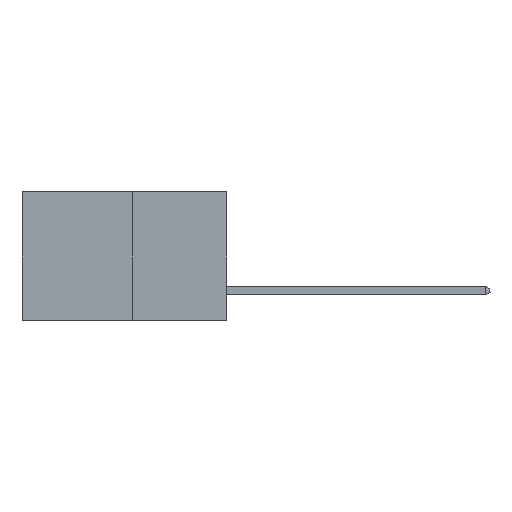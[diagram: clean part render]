
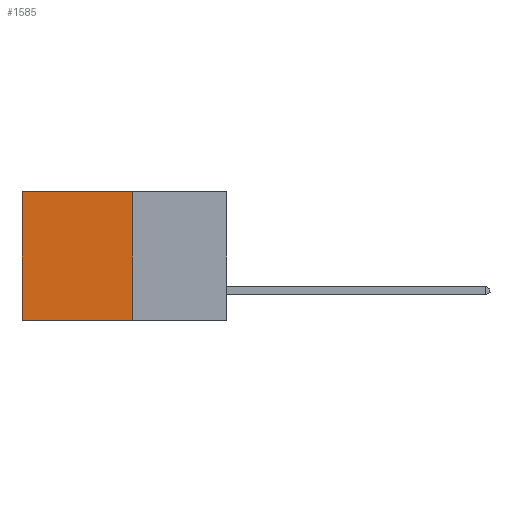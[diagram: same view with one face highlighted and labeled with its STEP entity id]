
A CAD part, left-side view. The second image highlights one B-rep face of the part: STEP entity #1585.
In plain terms, the highlighted planar face has unit normal (-1, 0, 0).
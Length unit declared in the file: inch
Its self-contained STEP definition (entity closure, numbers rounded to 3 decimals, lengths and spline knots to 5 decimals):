
#1541 = VERTEX_POINT ( 'NONE', #22558 ) ;
#1585 = ADVANCED_FACE ( 'NONE', ( #32372 ), #22675, .F. ) ;
#1615 = DIRECTION ( 'NONE',  ( 0., 0., -1. ) ) ;
#1715 = CARTESIAN_POINT ( 'NONE',  ( 0.277, 0.27, -0.37 ) ) ;
#4461 = VECTOR ( 'NONE', #7080, 39.37008 ) ;
#4482 = CARTESIAN_POINT ( 'NONE',  ( 0.277, 0.27, 0. ) ) ;
#4551 = CARTESIAN_POINT ( 'NONE',  ( 0.277, 0.27, -0.37 ) ) ;
#7023 = VECTOR ( 'NONE', #25033, 39.37008 ) ;
#7080 = DIRECTION ( 'NONE',  ( 0., 1., 0. ) ) ;
#8642 = VECTOR ( 'NONE', #26296, 39.37008 ) ;
#9455 = LINE ( 'NONE', #13396, #8642 ) ;
#9544 = VERTEX_POINT ( 'NONE', #17054 ) ;
#9885 = DIRECTION ( 'NONE',  ( 0., 0., -1. ) ) ;
#12544 = VECTOR ( 'NONE', #1615, 39.37008 ) ;
#12632 = VERTEX_POINT ( 'NONE', #32757 ) ;
#13396 = CARTESIAN_POINT ( 'NONE',  ( 0.277, 0.59, -0.37 ) ) ;
#16610 = VERTEX_POINT ( 'NONE', #22399 ) ;
#16974 = EDGE_CURVE ( 'NONE', #16610, #9544, #9455, .T. ) ;
#17054 = CARTESIAN_POINT ( 'NONE',  ( 0.277, 0.59, -0.37 ) ) ;
#17643 = ORIENTED_EDGE ( 'NONE', *, *, #25207, .F. ) ;
#18208 = LINE ( 'NONE', #4482, #4461 ) ;
#19407 = LINE ( 'NONE', #32525, #12544 ) ;
#21716 = EDGE_CURVE ( 'NONE', #1541, #16610, #18208, .T. ) ;
#22399 = CARTESIAN_POINT ( 'NONE',  ( 0.277, 0.59, 0. ) ) ;
#22558 = CARTESIAN_POINT ( 'NONE',  ( 0.277, 0.27, 0. ) ) ;
#22675 = PLANE ( 'NONE',  #30998 ) ;
#24269 = ORIENTED_EDGE ( 'NONE', *, *, #21716, .T. ) ;
#24292 = EDGE_LOOP ( 'NONE', ( #32522, #17643, #26681, #24269 ) ) ;
#25033 = DIRECTION ( 'NONE',  ( 0., 1., 0. ) ) ;
#25207 = EDGE_CURVE ( 'NONE', #12632, #9544, #27622, .T. ) ;
#25339 = DIRECTION ( 'NONE',  ( 1., 0., 0. ) ) ;
#26296 = DIRECTION ( 'NONE',  ( 0., 0., -1. ) ) ;
#26681 = ORIENTED_EDGE ( 'NONE', *, *, #30540, .F. ) ;
#27622 = LINE ( 'NONE', #1715, #7023 ) ;
#30540 = EDGE_CURVE ( 'NONE', #1541, #12632, #19407, .T. ) ;
#30998 = AXIS2_PLACEMENT_3D ( 'NONE', #4551, #25339, #9885 ) ;
#32372 = FACE_OUTER_BOUND ( 'NONE', #24292, .T. ) ;
#32522 = ORIENTED_EDGE ( 'NONE', *, *, #16974, .T. ) ;
#32525 = CARTESIAN_POINT ( 'NONE',  ( 0.277, 0.27, -0.37 ) ) ;
#32757 = CARTESIAN_POINT ( 'NONE',  ( 0.277, 0.27, -0.37 ) ) ;
